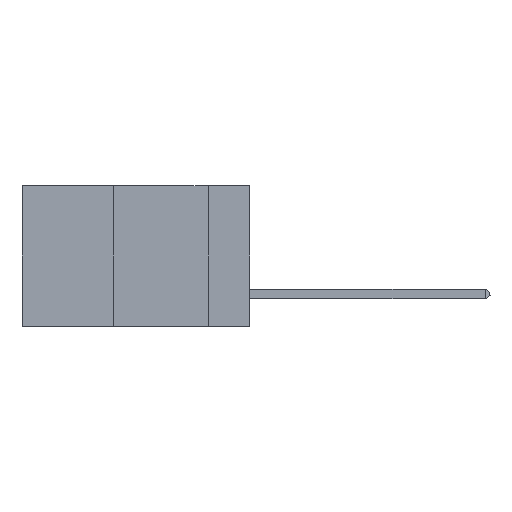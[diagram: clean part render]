
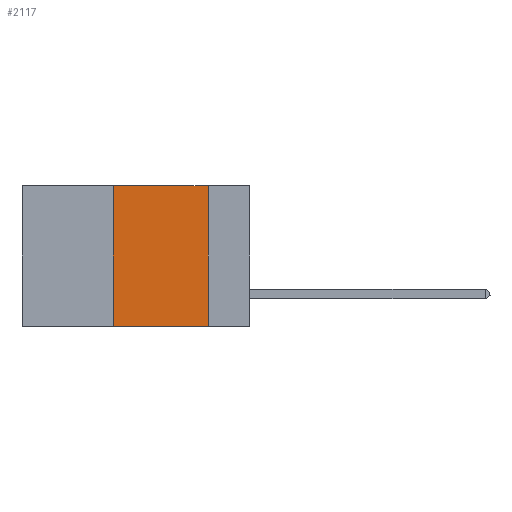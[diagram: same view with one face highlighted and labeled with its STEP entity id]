
A CAD part, left-side view. The second image highlights one B-rep face of the part: STEP entity #2117.
In plain terms, the highlighted planar face has unit normal (-1, 0, 0).
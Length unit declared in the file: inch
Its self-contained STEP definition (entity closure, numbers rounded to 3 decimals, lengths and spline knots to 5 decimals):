
#9 = ORIENTED_EDGE ( 'NONE', *, *, #1766, .F. ) ;
#98 = DIRECTION ( 'NONE',  ( 0., 0., -1. ) ) ;
#120 = ORIENTED_EDGE ( 'NONE', *, *, #4438, .T. ) ;
#427 = EDGE_CURVE ( 'NONE', #3325, #12062, #9383, .T. ) ;
#694 = EDGE_LOOP ( 'NONE', ( #9, #9606, #11282, #120 ) ) ;
#1766 = EDGE_CURVE ( 'NONE', #12062, #7687, #9689, .T. ) ;
#1940 = AXIS2_PLACEMENT_3D ( 'NONE', #6765, #7791, #98 ) ;
#1973 = DIRECTION ( 'NONE',  ( 0., -1., 0. ) ) ;
#2117 = ADVANCED_FACE ( 'NONE', ( #7004 ), #4799, .F. ) ;
#2337 = VECTOR ( 'NONE', #3575, 39.37008 ) ;
#2486 = CARTESIAN_POINT ( 'NONE',  ( 0., 0.36, 0. ) ) ;
#2935 = LINE ( 'NONE', #10062, #8679 ) ;
#3325 = VERTEX_POINT ( 'NONE', #2486 ) ;
#3575 = DIRECTION ( 'NONE',  ( 0., 0., 1. ) ) ;
#4405 = DIRECTION ( 'NONE',  ( 0., -1., 0. ) ) ;
#4438 = EDGE_CURVE ( 'NONE', #9722, #7687, #2935, .T. ) ;
#4799 = PLANE ( 'NONE',  #1940 ) ;
#5575 = CARTESIAN_POINT ( 'NONE',  ( 0., 0.36, 0. ) ) ;
#5958 = EDGE_CURVE ( 'NONE', #9722, #3325, #7771, .T. ) ;
#6335 = CARTESIAN_POINT ( 'NONE',  ( 0., 0.6, 0. ) ) ;
#6765 = CARTESIAN_POINT ( 'NONE',  ( 0., 0.6, 0. ) ) ;
#6874 = CARTESIAN_POINT ( 'NONE',  ( 0., 0.11, -0.37 ) ) ;
#7004 = FACE_OUTER_BOUND ( 'NONE', #694, .T. ) ;
#7019 = VECTOR ( 'NONE', #11733, 39.37008 ) ;
#7687 = VERTEX_POINT ( 'NONE', #6874 ) ;
#7771 = LINE ( 'NONE', #5575, #2337 ) ;
#7791 = DIRECTION ( 'NONE',  ( 1., 0., 0. ) ) ;
#8679 = VECTOR ( 'NONE', #1973, 39.37008 ) ;
#9383 = LINE ( 'NONE', #6335, #11906 ) ;
#9606 = ORIENTED_EDGE ( 'NONE', *, *, #427, .F. ) ;
#9689 = LINE ( 'NONE', #12720, #7019 ) ;
#9722 = VERTEX_POINT ( 'NONE', #12966 ) ;
#10062 = CARTESIAN_POINT ( 'NONE',  ( 0., 0.6, -0.37 ) ) ;
#11282 = ORIENTED_EDGE ( 'NONE', *, *, #5958, .F. ) ;
#11733 = DIRECTION ( 'NONE',  ( 0., 0., -1. ) ) ;
#11906 = VECTOR ( 'NONE', #4405, 39.37008 ) ;
#12062 = VERTEX_POINT ( 'NONE', #12255 ) ;
#12255 = CARTESIAN_POINT ( 'NONE',  ( 0., 0.11, 0. ) ) ;
#12720 = CARTESIAN_POINT ( 'NONE',  ( 0., 0.11, 0. ) ) ;
#12966 = CARTESIAN_POINT ( 'NONE',  ( 0., 0.36, -0.37 ) ) ;
